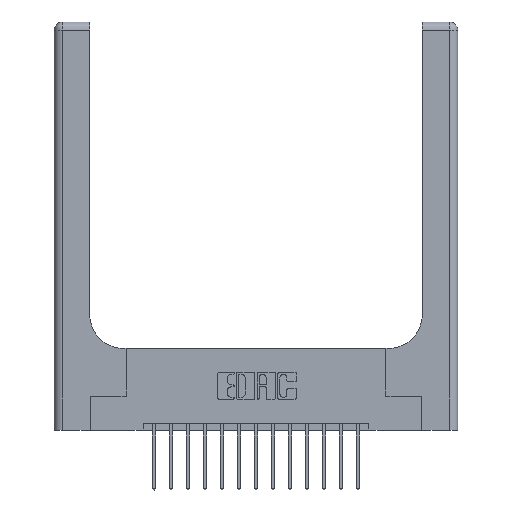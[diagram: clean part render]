
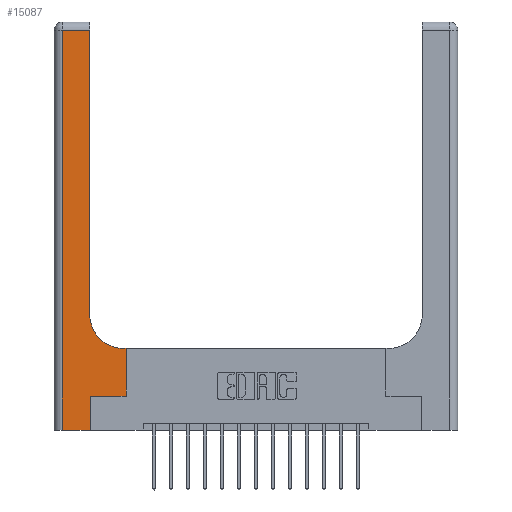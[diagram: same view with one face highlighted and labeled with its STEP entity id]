
A CAD part, top view. The second image highlights one B-rep face of the part: STEP entity #15087.
In plain terms, the highlighted planar face has unit normal (0, 0, 1).
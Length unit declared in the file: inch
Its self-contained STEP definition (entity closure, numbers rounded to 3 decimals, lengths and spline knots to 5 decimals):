
#362 = EDGE_CURVE ( 'NONE', #14967, #9764, #16619, .T. ) ;
#747 = ORIENTED_EDGE ( 'NONE', *, *, #9039, .T. ) ;
#788 = VECTOR ( 'NONE', #12873, 39.37008 ) ;
#1014 = VERTEX_POINT ( 'NONE', #2434 ) ;
#1520 = CARTESIAN_POINT ( 'NONE',  ( 0.06, 2.94, 0.37 ) ) ;
#1701 = VERTEX_POINT ( 'NONE', #3214 ) ;
#1833 = EDGE_CURVE ( 'NONE', #9764, #7601, #10045, .T. ) ;
#1945 = EDGE_LOOP ( 'NONE', ( #747, #14260, #5399, #11178, #14778, #9168, #9217, #3628, #3869 ) ) ;
#2041 = DIRECTION ( 'NONE',  ( -1., 0., 0. ) ) ;
#2073 = AXIS2_PLACEMENT_3D ( 'NONE', #11006, #3784, #2818 ) ;
#2130 = VECTOR ( 'NONE', #5553, 39.37008 ) ;
#2434 = CARTESIAN_POINT ( 'NONE',  ( 0.06, 0., 0.37 ) ) ;
#2474 = CARTESIAN_POINT ( 'NONE',  ( 0.26, 2.94, 0.37 ) ) ;
#2492 = CARTESIAN_POINT ( 'NONE',  ( 0.26, 3., 0.37 ) ) ;
#2802 = EDGE_CURVE ( 'NONE', #7601, #7280, #14659, .T. ) ;
#2818 = DIRECTION ( 'NONE',  ( 1., 0., 0. ) ) ;
#2841 = CARTESIAN_POINT ( 'NONE',  ( 0.528, 0.25, 0.37 ) ) ;
#3214 = CARTESIAN_POINT ( 'NONE',  ( 0.26, 0.85, 0.37 ) ) ;
#3291 = VERTEX_POINT ( 'NONE', #1520 ) ;
#3628 = ORIENTED_EDGE ( 'NONE', *, *, #2802, .T. ) ;
#3673 = CIRCLE ( 'NONE', #2073, 0.25 ) ;
#3784 = DIRECTION ( 'NONE',  ( 0., 0., -1. ) ) ;
#3869 = ORIENTED_EDGE ( 'NONE', *, *, #11170, .T. ) ;
#3958 = CARTESIAN_POINT ( 'NONE',  ( 0.265, 0., 0.37 ) ) ;
#4182 = CARTESIAN_POINT ( 'NONE',  ( 0.26, 0.6, 0.37 ) ) ;
#4342 = EDGE_CURVE ( 'NONE', #1014, #12099, #13141, .T. ) ;
#4570 = VECTOR ( 'NONE', #7346, 39.37008 ) ;
#5399 = ORIENTED_EDGE ( 'NONE', *, *, #13332, .T. ) ;
#5553 = DIRECTION ( 'NONE',  ( 0., 1., 0. ) ) ;
#6008 = VECTOR ( 'NONE', #14181, 39.37008 ) ;
#6860 = LINE ( 'NONE', #8730, #12642 ) ;
#7049 = LINE ( 'NONE', #7803, #16809 ) ;
#7280 = VERTEX_POINT ( 'NONE', #10501 ) ;
#7346 = DIRECTION ( 'NONE',  ( -1., 0., 0. ) ) ;
#7483 = CARTESIAN_POINT ( 'NONE',  ( 0., 3., 0.37 ) ) ;
#7601 = VERTEX_POINT ( 'NONE', #17558 ) ;
#7654 = VECTOR ( 'NONE', #9864, 39.37008 ) ;
#7803 = CARTESIAN_POINT ( 'NONE',  ( 0.06, 3., 0.37 ) ) ;
#7864 = DIRECTION ( 'NONE',  ( 0., -1., 0. ) ) ;
#8730 = CARTESIAN_POINT ( 'NONE',  ( 0.265, 0., 0.37 ) ) ;
#8881 = AXIS2_PLACEMENT_3D ( 'NONE', #7483, #16966, #2041 ) ;
#9039 = EDGE_CURVE ( 'NONE', #1701, #13411, #15882, .T. ) ;
#9168 = ORIENTED_EDGE ( 'NONE', *, *, #362, .T. ) ;
#9217 = ORIENTED_EDGE ( 'NONE', *, *, #1833, .T. ) ;
#9277 = DIRECTION ( 'NONE',  ( 0., 1., 0. ) ) ;
#9672 = CARTESIAN_POINT ( 'NONE',  ( 0., 2.94, 0.37 ) ) ;
#9684 = DIRECTION ( 'NONE',  ( 0., 1., 0. ) ) ;
#9764 = VERTEX_POINT ( 'NONE', #15929 ) ;
#9864 = DIRECTION ( 'NONE',  ( -1., 0., 0. ) ) ;
#9954 = EDGE_CURVE ( 'NONE', #13411, #3291, #12478, .T. ) ;
#10045 = LINE ( 'NONE', #2841, #2130 ) ;
#10501 = CARTESIAN_POINT ( 'NONE',  ( 0.51, 0.6, 0.37 ) ) ;
#11006 = CARTESIAN_POINT ( 'NONE',  ( 0.51, 0.85, 0.37 ) ) ;
#11170 = EDGE_CURVE ( 'NONE', #7280, #1701, #3673, .T. ) ;
#11178 = ORIENTED_EDGE ( 'NONE', *, *, #4342, .T. ) ;
#11882 = VECTOR ( 'NONE', #9684, 39.37008 ) ;
#12099 = VERTEX_POINT ( 'NONE', #3958 ) ;
#12478 = LINE ( 'NONE', #9672, #4570 ) ;
#12600 = EDGE_CURVE ( 'NONE', #12099, #14967, #6860, .T. ) ;
#12628 = CARTESIAN_POINT ( 'NONE',  ( 0.265, 0.25, 0.37 ) ) ;
#12642 = VECTOR ( 'NONE', #9277, 39.37008 ) ;
#12807 = CARTESIAN_POINT ( 'NONE',  ( 0.265, 0.25, 0.37 ) ) ;
#12873 = DIRECTION ( 'NONE',  ( 1., 0., 0. ) ) ;
#12961 = FACE_OUTER_BOUND ( 'NONE', #1945, .T. ) ;
#13141 = LINE ( 'NONE', #15807, #788 ) ;
#13332 = EDGE_CURVE ( 'NONE', #3291, #1014, #7049, .T. ) ;
#13411 = VERTEX_POINT ( 'NONE', #2474 ) ;
#14177 = PLANE ( 'NONE',  #8881 ) ;
#14181 = DIRECTION ( 'NONE',  ( 1., 0., 0. ) ) ;
#14260 = ORIENTED_EDGE ( 'NONE', *, *, #9954, .T. ) ;
#14659 = LINE ( 'NONE', #4182, #7654 ) ;
#14778 = ORIENTED_EDGE ( 'NONE', *, *, #12600, .T. ) ;
#14967 = VERTEX_POINT ( 'NONE', #12628 ) ;
#15087 = ADVANCED_FACE ( 'NONE', ( #12961 ), #14177, .F. ) ;
#15807 = CARTESIAN_POINT ( 'NONE',  ( 0., 0., 0.37 ) ) ;
#15882 = LINE ( 'NONE', #2492, #11882 ) ;
#15929 = CARTESIAN_POINT ( 'NONE',  ( 0.528, 0.25, 0.37 ) ) ;
#16619 = LINE ( 'NONE', #12807, #6008 ) ;
#16809 = VECTOR ( 'NONE', #7864, 39.37008 ) ;
#16966 = DIRECTION ( 'NONE',  ( 0., 0., -1. ) ) ;
#17558 = CARTESIAN_POINT ( 'NONE',  ( 0.528, 0.6, 0.37 ) ) ;
